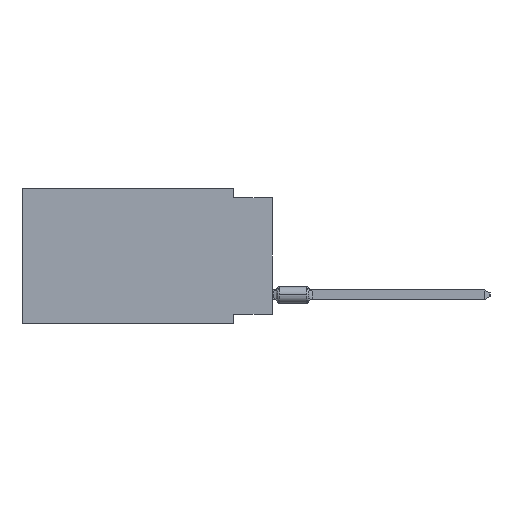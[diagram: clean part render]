
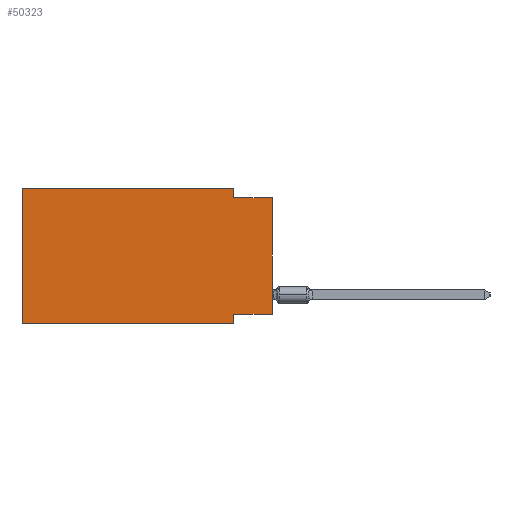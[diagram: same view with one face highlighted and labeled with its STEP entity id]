
A CAD part, left-side view. The second image highlights one B-rep face of the part: STEP entity #50323.
In plain terms, the highlighted planar face has unit normal (-1, 0, 0).
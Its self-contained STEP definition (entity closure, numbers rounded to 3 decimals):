
#423 = CARTESIAN_POINT ( 'NONE',  ( 0., 2.54, -0.635 ) ) ;
#459 = EDGE_CURVE ( 'NONE', #30237, #5230, #4423, .T. ) ;
#907 = CARTESIAN_POINT ( 'NONE',  ( 0., 2.54, -8.255 ) ) ;
#1480 = ORIENTED_EDGE ( 'NONE', *, *, #459, .F. ) ;
#3121 = CARTESIAN_POINT ( 'NONE',  ( 0., 2.54, -8.89 ) ) ;
#3709 = VECTOR ( 'NONE', #11233, 1000. ) ;
#4104 = CARTESIAN_POINT ( 'NONE',  ( 0., 0., -0.635 ) ) ;
#4289 = VERTEX_POINT ( 'NONE', #42944 ) ;
#4423 = LINE ( 'NONE', #16638, #27916 ) ;
#5230 = VERTEX_POINT ( 'NONE', #35844 ) ;
#7698 = ORIENTED_EDGE ( 'NONE', *, *, #27007, .F. ) ;
#9213 = VECTOR ( 'NONE', #25043, 1000. ) ;
#9861 = ORIENTED_EDGE ( 'NONE', *, *, #49215, .F. ) ;
#10870 = EDGE_CURVE ( 'NONE', #32082, #36350, #48549, .T. ) ;
#11233 = DIRECTION ( 'NONE',  ( 0., -1., 0. ) ) ;
#11430 = LINE ( 'NONE', #27985, #24397 ) ;
#11697 = AXIS2_PLACEMENT_3D ( 'NONE', #45123, #19864, #23688 ) ;
#11786 = CARTESIAN_POINT ( 'NONE',  ( 0., 16.383, -8.89 ) ) ;
#13843 = CARTESIAN_POINT ( 'NONE',  ( 0., 0., -8.255 ) ) ;
#15468 = VECTOR ( 'NONE', #18474, 1000. ) ;
#16349 = CARTESIAN_POINT ( 'NONE',  ( 0., 16.383, 0. ) ) ;
#16638 = CARTESIAN_POINT ( 'NONE',  ( 0., 16.383, 0. ) ) ;
#18474 = DIRECTION ( 'NONE',  ( 0., 0., -1. ) ) ;
#18998 = CARTESIAN_POINT ( 'NONE',  ( 0., 2.54, 0. ) ) ;
#19657 = DIRECTION ( 'NONE',  ( 0., 0., -1. ) ) ;
#19864 = DIRECTION ( 'NONE',  ( 1., 0., 0. ) ) ;
#20215 = VECTOR ( 'NONE', #19657, 1000. ) ;
#20652 = EDGE_LOOP ( 'NONE', ( #32247, #22393, #7698, #1480, #39196, #41350, #9861, #28398 ) ) ;
#20722 = VERTEX_POINT ( 'NONE', #11786 ) ;
#22393 = ORIENTED_EDGE ( 'NONE', *, *, #23048, .F. ) ;
#22672 = VECTOR ( 'NONE', #25810, 1000. ) ;
#22920 = VECTOR ( 'NONE', #44208, 1000. ) ;
#23048 = EDGE_CURVE ( 'NONE', #48293, #38908, #35674, .T. ) ;
#23688 = DIRECTION ( 'NONE',  ( 0., 0., -1. ) ) ;
#24397 = VECTOR ( 'NONE', #53229, 1000. ) ;
#25043 = DIRECTION ( 'NONE',  ( 0., 0., 1. ) ) ;
#25810 = DIRECTION ( 'NONE',  ( 0., 0., 1. ) ) ;
#26281 = CARTESIAN_POINT ( 'NONE',  ( 0., 0., -0.635 ) ) ;
#27007 = EDGE_CURVE ( 'NONE', #5230, #48293, #35841, .T. ) ;
#27642 = CARTESIAN_POINT ( 'NONE',  ( 0., 0., -8.255 ) ) ;
#27916 = VECTOR ( 'NONE', #38073, 1000. ) ;
#27985 = CARTESIAN_POINT ( 'NONE',  ( 0., 16.383, -8.89 ) ) ;
#28398 = ORIENTED_EDGE ( 'NONE', *, *, #10870, .F. ) ;
#28562 = PLANE ( 'NONE',  #11697 ) ;
#29676 = LINE ( 'NONE', #51108, #9213 ) ;
#30237 = VERTEX_POINT ( 'NONE', #16349 ) ;
#32082 = VERTEX_POINT ( 'NONE', #13843 ) ;
#32247 = ORIENTED_EDGE ( 'NONE', *, *, #51728, .T. ) ;
#33966 = LINE ( 'NONE', #38574, #22672 ) ;
#35674 = LINE ( 'NONE', #26281, #3709 ) ;
#35841 = LINE ( 'NONE', #18998, #15468 ) ;
#35844 = CARTESIAN_POINT ( 'NONE',  ( 0., 2.54, 0. ) ) ;
#36350 = VERTEX_POINT ( 'NONE', #907 ) ;
#37032 = LINE ( 'NONE', #3121, #20215 ) ;
#38073 = DIRECTION ( 'NONE',  ( 0., -1., 0. ) ) ;
#38574 = CARTESIAN_POINT ( 'NONE',  ( 0., 16.383, 0. ) ) ;
#38901 = EDGE_CURVE ( 'NONE', #20722, #4289, #11430, .T. ) ;
#38908 = VERTEX_POINT ( 'NONE', #4104 ) ;
#39023 = EDGE_CURVE ( 'NONE', #20722, #30237, #33966, .T. ) ;
#39196 = ORIENTED_EDGE ( 'NONE', *, *, #39023, .F. ) ;
#41350 = ORIENTED_EDGE ( 'NONE', *, *, #38901, .T. ) ;
#42944 = CARTESIAN_POINT ( 'NONE',  ( 0., 2.54, -8.89 ) ) ;
#44208 = DIRECTION ( 'NONE',  ( 0., 1., 0. ) ) ;
#44855 = FACE_OUTER_BOUND ( 'NONE', #20652, .T. ) ;
#45123 = CARTESIAN_POINT ( 'NONE',  ( 0., 16.383, 0. ) ) ;
#48293 = VERTEX_POINT ( 'NONE', #423 ) ;
#48549 = LINE ( 'NONE', #27642, #22920 ) ;
#49215 = EDGE_CURVE ( 'NONE', #36350, #4289, #37032, .T. ) ;
#50323 = ADVANCED_FACE ( 'NONE', ( #44855 ), #28562, .F. ) ;
#51108 = CARTESIAN_POINT ( 'NONE',  ( 0., 0., 0. ) ) ;
#51728 = EDGE_CURVE ( 'NONE', #32082, #38908, #29676, .T. ) ;
#53229 = DIRECTION ( 'NONE',  ( 0., -1., 0. ) ) ;
